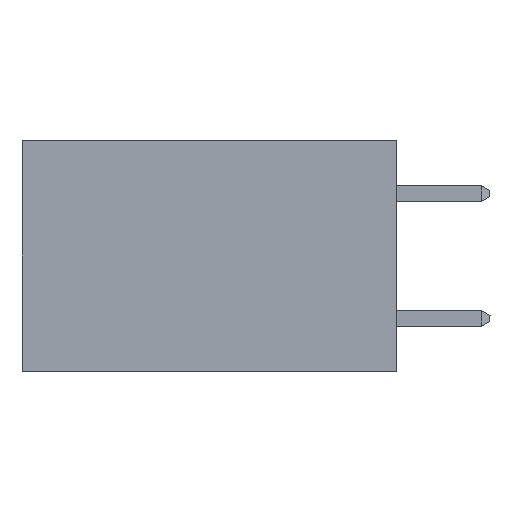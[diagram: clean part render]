
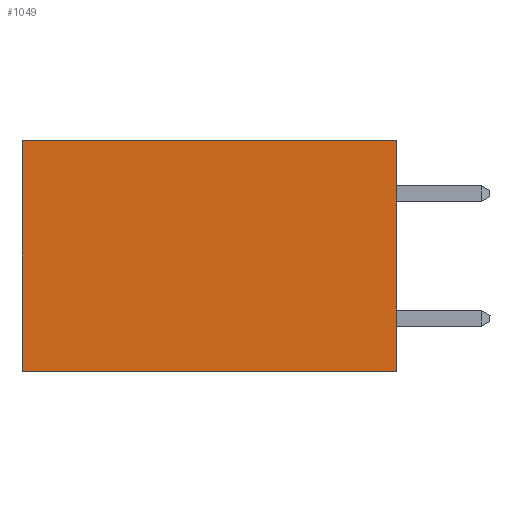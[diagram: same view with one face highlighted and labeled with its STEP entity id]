
A CAD part, left-side view. The second image highlights one B-rep face of the part: STEP entity #1049.
In plain terms, the highlighted planar face has unit normal (-1, 0, 0).
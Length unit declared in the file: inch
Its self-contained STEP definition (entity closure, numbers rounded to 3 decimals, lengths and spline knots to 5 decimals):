
#719 = FACE_OUTER_BOUND ( 'NONE', #18819, .T. ) ;
#1049 = ADVANCED_FACE ( 'NONE', ( #719 ), #16601, .F. ) ;
#1131 = LINE ( 'NONE', #6873, #16257 ) ;
#2436 = DIRECTION ( 'NONE',  ( 0., 0., -1. ) ) ;
#2958 = DIRECTION ( 'NONE',  ( 0., 1., 0. ) ) ;
#3018 = EDGE_CURVE ( 'NONE', #15711, #20146, #26987, .T. ) ;
#3256 = CARTESIAN_POINT ( 'NONE',  ( 0.298, 0.6, -0.37 ) ) ;
#3751 = CARTESIAN_POINT ( 'NONE',  ( 0.298, 0.6, 0. ) ) ;
#5040 = EDGE_CURVE ( 'NONE', #22395, #15711, #11036, .T. ) ;
#5167 = CARTESIAN_POINT ( 'NONE',  ( 0.298, 0., 0. ) ) ;
#5914 = DIRECTION ( 'NONE',  ( 0., 1., 0. ) ) ;
#6134 = DIRECTION ( 'NONE',  ( 0., 0., -1. ) ) ;
#6873 = CARTESIAN_POINT ( 'NONE',  ( 0.298, 0.6, 0. ) ) ;
#8248 = DIRECTION ( 'NONE',  ( 1., 0., 0. ) ) ;
#8634 = VERTEX_POINT ( 'NONE', #3751 ) ;
#11036 = LINE ( 'NONE', #26439, #24443 ) ;
#11986 = ORIENTED_EDGE ( 'NONE', *, *, #20147, .T. ) ;
#12059 = ORIENTED_EDGE ( 'NONE', *, *, #3018, .F. ) ;
#12991 = LINE ( 'NONE', #5167, #25010 ) ;
#14592 = CARTESIAN_POINT ( 'NONE',  ( 0.298, 0., 0. ) ) ;
#15640 = CARTESIAN_POINT ( 'NONE',  ( 0.298, 0., -0.37 ) ) ;
#15711 = VERTEX_POINT ( 'NONE', #15640 ) ;
#16257 = VECTOR ( 'NONE', #22225, 39.37008 ) ;
#16601 = PLANE ( 'NONE',  #21501 ) ;
#18819 = EDGE_LOOP ( 'NONE', ( #25779, #12059, #24089, #11986 ) ) ;
#20146 = VERTEX_POINT ( 'NONE', #3256 ) ;
#20147 = EDGE_CURVE ( 'NONE', #22395, #8634, #12991, .T. ) ;
#20424 = VECTOR ( 'NONE', #5914, 39.37008 ) ;
#21501 = AXIS2_PLACEMENT_3D ( 'NONE', #14592, #8248, #6134 ) ;
#22225 = DIRECTION ( 'NONE',  ( 0., 0., -1. ) ) ;
#22395 = VERTEX_POINT ( 'NONE', #23586 ) ;
#23586 = CARTESIAN_POINT ( 'NONE',  ( 0.298, 0., 0. ) ) ;
#24089 = ORIENTED_EDGE ( 'NONE', *, *, #5040, .F. ) ;
#24443 = VECTOR ( 'NONE', #2436, 39.37008 ) ;
#25010 = VECTOR ( 'NONE', #2958, 39.37008 ) ;
#25779 = ORIENTED_EDGE ( 'NONE', *, *, #27185, .T. ) ;
#26439 = CARTESIAN_POINT ( 'NONE',  ( 0.298, 0., 0. ) ) ;
#26987 = LINE ( 'NONE', #27803, #20424 ) ;
#27185 = EDGE_CURVE ( 'NONE', #8634, #20146, #1131, .T. ) ;
#27803 = CARTESIAN_POINT ( 'NONE',  ( 0.298, 0., -0.37 ) ) ;
